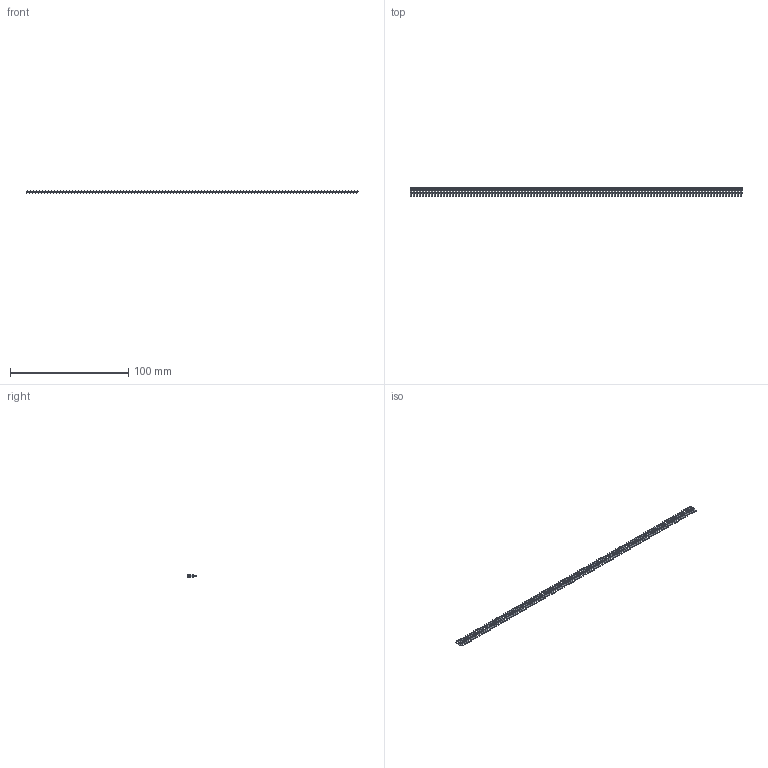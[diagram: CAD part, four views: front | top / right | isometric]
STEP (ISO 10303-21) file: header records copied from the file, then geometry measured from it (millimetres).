
FILE_DESCRIPTION (( 'STEP AP203' ), '1' );
FILE_NAME ('106-111-253-100.STEP', '2020-04-16T23:36:28', ( '' ), ( '' ), 'SwSTEP 2.0', 'SolidWorks 2016', '' );
FILE_SCHEMA (( 'CONFIG_CONTROL_DESIGN' ));
Length unit declared in the file: inch
Products named in the file (2): 106-111-253-100; 100-290-001_100-290-253
Assembly tree (111 placements, depth 2):
  106-111-253-100
    100-290-001_100-290-253  x111
Bounding box: 281.2 x 7.62 x 1.8 mm (x, y, z)
Volume: 612.5 mm3; surface area: 3819.2 mm2
Topology: 111 solids, 111 shells, 2220 faces, 5994 edges, 3996 vertices
Faces by surface type: plane 2109, cylinder 111
Entity records: 4340 total; most frequent: DIRECTION 324, LOCAL_TIME 232, CALENDAR_DATE 232, COORDINATED_UNIVERSAL_TIME_OFFSET 232, DATE_AND_TIME 232, CARTESIAN_POINT 224, AXIS2_PLACEMENT_3D 136, PERSON_AND_ORGANIZATION 127
